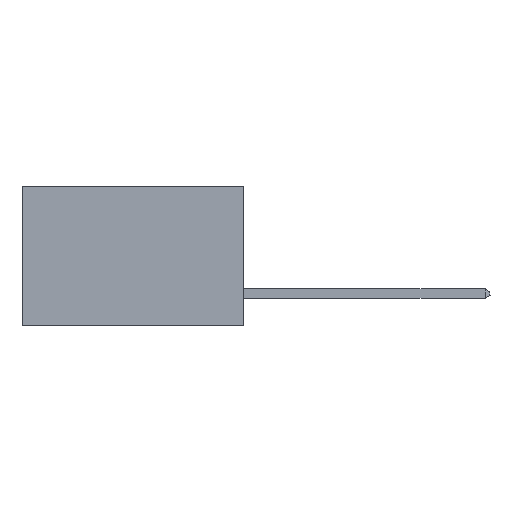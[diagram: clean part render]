
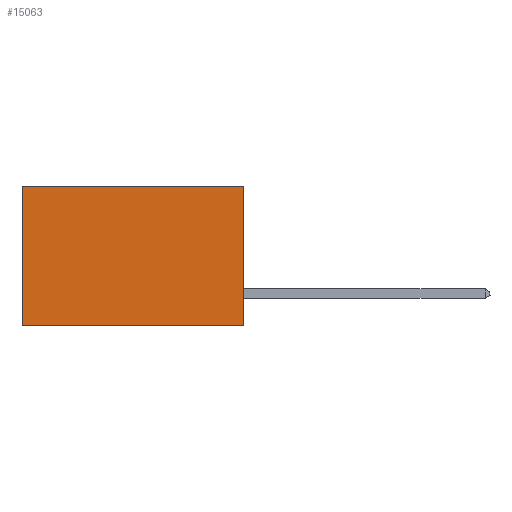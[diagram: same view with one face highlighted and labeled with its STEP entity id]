
A CAD part, left-side view. The second image highlights one B-rep face of the part: STEP entity #15063.
In plain terms, the highlighted planar face has unit normal (-1, 0, 0).
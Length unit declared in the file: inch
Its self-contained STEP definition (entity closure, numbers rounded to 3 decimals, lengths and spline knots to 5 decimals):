
#676 = EDGE_CURVE ( 'NONE', #3567, #4638, #6036, .T. ) ;
#1286 = ORIENTED_EDGE ( 'NONE', *, *, #8990, .F. ) ;
#1404 = VECTOR ( 'NONE', #8960, 39.37008 ) ;
#2476 = VECTOR ( 'NONE', #16205, 39.37008 ) ;
#2597 = ORIENTED_EDGE ( 'NONE', *, *, #14042, .F. ) ;
#3567 = VERTEX_POINT ( 'NONE', #13396 ) ;
#4516 = VERTEX_POINT ( 'NONE', #11112 ) ;
#4638 = VERTEX_POINT ( 'NONE', #14994 ) ;
#5103 = CARTESIAN_POINT ( 'NONE',  ( 0.277, 0., -0.37 ) ) ;
#5330 = CARTESIAN_POINT ( 'NONE',  ( 0.277, 0., -0.37 ) ) ;
#6036 = LINE ( 'NONE', #12589, #16051 ) ;
#6049 = DIRECTION ( 'NONE',  ( 1., 0., 0. ) ) ;
#6900 = EDGE_LOOP ( 'NONE', ( #12528, #1286, #2597, #12217 ) ) ;
#7116 = LINE ( 'NONE', #14891, #13968 ) ;
#8960 = DIRECTION ( 'NONE',  ( 0., 0., -1. ) ) ;
#8990 = EDGE_CURVE ( 'NONE', #11145, #4516, #7116, .T. ) ;
#9112 = EDGE_CURVE ( 'NONE', #4638, #4516, #15853, .T. ) ;
#9480 = AXIS2_PLACEMENT_3D ( 'NONE', #11530, #6049, #15600 ) ;
#11112 = CARTESIAN_POINT ( 'NONE',  ( 0.277, 0.59, -0.37 ) ) ;
#11145 = VERTEX_POINT ( 'NONE', #5103 ) ;
#11503 = CARTESIAN_POINT ( 'NONE',  ( 0.277, 0.59, -0.37 ) ) ;
#11530 = CARTESIAN_POINT ( 'NONE',  ( 0.277, 0., -0.37 ) ) ;
#12217 = ORIENTED_EDGE ( 'NONE', *, *, #676, .T. ) ;
#12528 = ORIENTED_EDGE ( 'NONE', *, *, #9112, .T. ) ;
#12589 = CARTESIAN_POINT ( 'NONE',  ( 0.277, 0., 0. ) ) ;
#13085 = FACE_OUTER_BOUND ( 'NONE', #6900, .T. ) ;
#13396 = CARTESIAN_POINT ( 'NONE',  ( 0.277, 0., 0. ) ) ;
#13968 = VECTOR ( 'NONE', #14808, 39.37008 ) ;
#14042 = EDGE_CURVE ( 'NONE', #3567, #11145, #16467, .T. ) ;
#14253 = PLANE ( 'NONE',  #9480 ) ;
#14808 = DIRECTION ( 'NONE',  ( 0., 1., 0. ) ) ;
#14891 = CARTESIAN_POINT ( 'NONE',  ( 0.277, 0., -0.37 ) ) ;
#14994 = CARTESIAN_POINT ( 'NONE',  ( 0.277, 0.59, 0. ) ) ;
#15063 = ADVANCED_FACE ( 'NONE', ( #13085 ), #14253, .F. ) ;
#15089 = DIRECTION ( 'NONE',  ( 0., 1., 0. ) ) ;
#15600 = DIRECTION ( 'NONE',  ( 0., 0., -1. ) ) ;
#15853 = LINE ( 'NONE', #11503, #1404 ) ;
#16051 = VECTOR ( 'NONE', #15089, 39.37008 ) ;
#16205 = DIRECTION ( 'NONE',  ( 0., 0., -1. ) ) ;
#16467 = LINE ( 'NONE', #5330, #2476 ) ;
